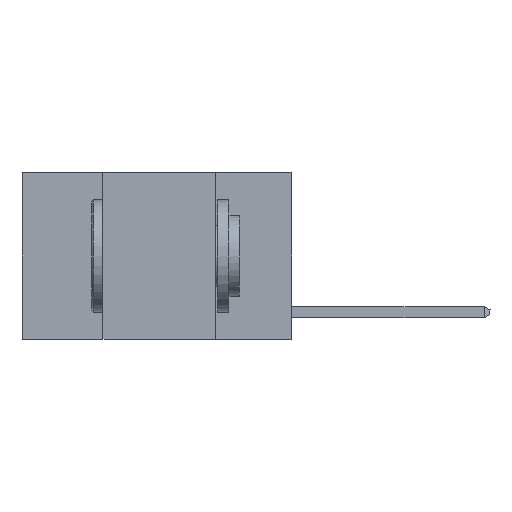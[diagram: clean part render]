
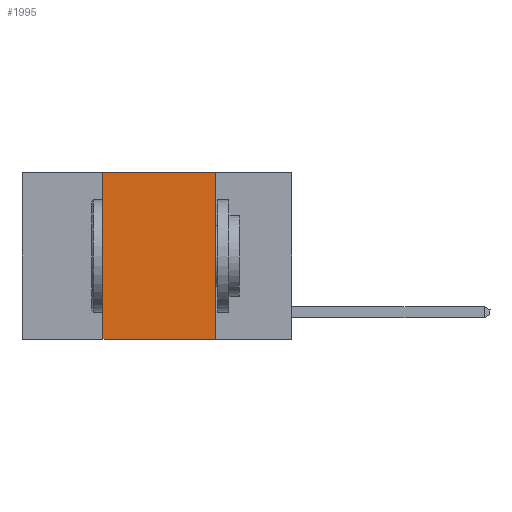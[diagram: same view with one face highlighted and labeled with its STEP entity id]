
A CAD part, left-side view. The second image highlights one B-rep face of the part: STEP entity #1995.
In plain terms, the highlighted planar face has unit normal (-1, 0, 0).
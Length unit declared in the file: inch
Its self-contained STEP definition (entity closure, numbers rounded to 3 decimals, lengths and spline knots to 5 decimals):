
#1292 = DIRECTION ( 'NONE',  ( 0., -1., 0. ) ) ;
#1652 = EDGE_CURVE ( 'NONE', #15296, #7459, #18208, .T. ) ;
#1995 = ADVANCED_FACE ( 'NONE', ( #20749 ), #23106, .F. ) ;
#2502 = VECTOR ( 'NONE', #2642, 39.37008 ) ;
#2524 = EDGE_CURVE ( 'NONE', #15296, #4615, #3184, .T. ) ;
#2529 = VECTOR ( 'NONE', #12623, 39.37008 ) ;
#2642 = DIRECTION ( 'NONE',  ( 0., 0., -1. ) ) ;
#3079 = ORIENTED_EDGE ( 'NONE', *, *, #13191, .F. ) ;
#3184 = LINE ( 'NONE', #12791, #2529 ) ;
#3732 = ORIENTED_EDGE ( 'NONE', *, *, #1652, .T. ) ;
#4569 = CARTESIAN_POINT ( 'NONE',  ( 0., 0.17, 0. ) ) ;
#4615 = VERTEX_POINT ( 'NONE', #19324 ) ;
#4654 = CARTESIAN_POINT ( 'NONE',  ( 0., 0.17, 0. ) ) ;
#5576 = CARTESIAN_POINT ( 'NONE',  ( 0., 0.42, -0.37 ) ) ;
#7314 = CARTESIAN_POINT ( 'NONE',  ( 0., 0.6, 0. ) ) ;
#7337 = DIRECTION ( 'NONE',  ( 0., -1., 0. ) ) ;
#7459 = VERTEX_POINT ( 'NONE', #20359 ) ;
#7971 = LINE ( 'NONE', #4654, #2502 ) ;
#9429 = EDGE_CURVE ( 'NONE', #14829, #7459, #7971, .T. ) ;
#11055 = DIRECTION ( 'NONE',  ( 0., 0., -1. ) ) ;
#11139 = DIRECTION ( 'NONE',  ( 1., 0., 0. ) ) ;
#11734 = CARTESIAN_POINT ( 'NONE',  ( 0., 0.6, -0.37 ) ) ;
#12623 = DIRECTION ( 'NONE',  ( 0., 0., 1. ) ) ;
#12791 = CARTESIAN_POINT ( 'NONE',  ( 0., 0.42, 0. ) ) ;
#12819 = VECTOR ( 'NONE', #1292, 39.37008 ) ;
#13191 = EDGE_CURVE ( 'NONE', #4615, #14829, #15682, .T. ) ;
#13316 = ORIENTED_EDGE ( 'NONE', *, *, #9429, .F. ) ;
#13942 = ORIENTED_EDGE ( 'NONE', *, *, #2524, .F. ) ;
#14829 = VERTEX_POINT ( 'NONE', #4569 ) ;
#15296 = VERTEX_POINT ( 'NONE', #5576 ) ;
#15682 = LINE ( 'NONE', #17462, #16304 ) ;
#16304 = VECTOR ( 'NONE', #7337, 39.37008 ) ;
#16639 = AXIS2_PLACEMENT_3D ( 'NONE', #7314, #11139, #11055 ) ;
#17462 = CARTESIAN_POINT ( 'NONE',  ( 0., 0.6, 0. ) ) ;
#17594 = EDGE_LOOP ( 'NONE', ( #13316, #3079, #13942, #3732 ) ) ;
#18208 = LINE ( 'NONE', #11734, #12819 ) ;
#19324 = CARTESIAN_POINT ( 'NONE',  ( 0., 0.42, 0. ) ) ;
#20359 = CARTESIAN_POINT ( 'NONE',  ( 0., 0.17, -0.37 ) ) ;
#20749 = FACE_OUTER_BOUND ( 'NONE', #17594, .T. ) ;
#23106 = PLANE ( 'NONE',  #16639 ) ;
